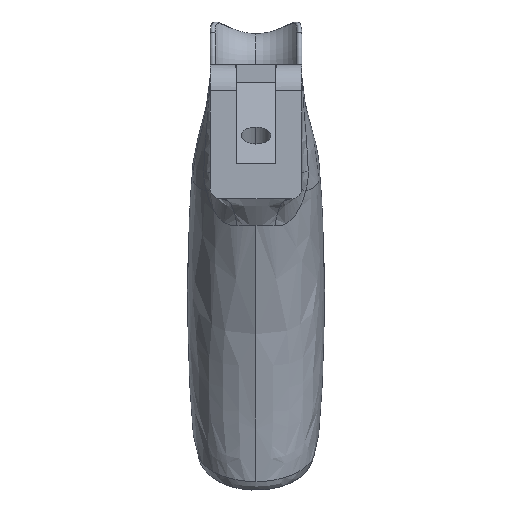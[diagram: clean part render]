
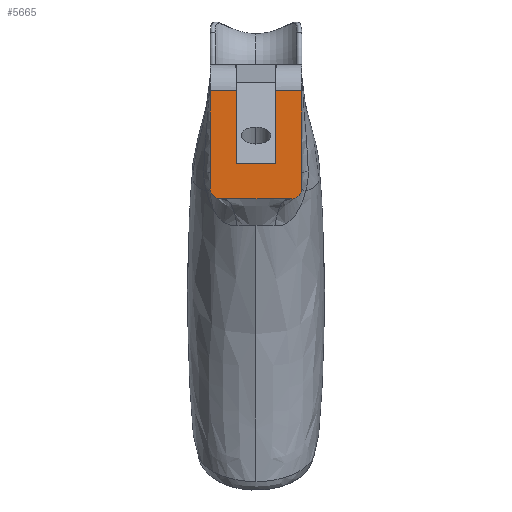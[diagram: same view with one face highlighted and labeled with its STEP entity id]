
A CAD part, top view. The second image highlights one B-rep face of the part: STEP entity #5665.
In plain terms, the highlighted planar face has unit normal (0, 0, 1).
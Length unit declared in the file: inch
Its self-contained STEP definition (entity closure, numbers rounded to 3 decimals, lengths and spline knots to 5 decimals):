
#47 = VERTEX_POINT ( 'NONE', #6501 ) ;
#377 = ORIENTED_EDGE ( 'NONE', *, *, #3790, .T. ) ;
#420 = DIRECTION ( 'NONE',  ( 0., 0., -1. ) ) ;
#441 = CARTESIAN_POINT ( 'NONE',  ( 0.1875, -0.25, 0. ) ) ;
#486 = CARTESIAN_POINT ( 'NONE',  ( 0.4375, -1.2789, 0. ) ) ;
#601 = VERTEX_POINT ( 'NONE', #441 ) ;
#726 = CARTESIAN_POINT ( 'NONE',  ( -0.3375, -1.2789, 0. ) ) ;
#776 = EDGE_CURVE ( 'NONE', #3794, #4979, #1841, .T. ) ;
#785 = EDGE_CURVE ( 'NONE', #3794, #4876, #6398, .T. ) ;
#873 = VERTEX_POINT ( 'NONE', #4419 ) ;
#920 = EDGE_LOOP ( 'NONE', ( #2350, #3677, #5511, #1936, #3274, #3456, #5523, #2167, #377, #1295 ) ) ;
#968 = CARTESIAN_POINT ( 'NONE',  ( 0.4375, -0.25, 0. ) ) ;
#1002 = LINE ( 'NONE', #2136, #7132 ) ;
#1037 = CARTESIAN_POINT ( 'NONE',  ( -0.1875, -0.94, 0. ) ) ;
#1239 = CARTESIAN_POINT ( 'NONE',  ( 0.4375, -0.25, 0. ) ) ;
#1260 = CARTESIAN_POINT ( 'NONE',  ( 0.4375, -1.1789, 0. ) ) ;
#1295 = ORIENTED_EDGE ( 'NONE', *, *, #1560, .T. ) ;
#1520 = VERTEX_POINT ( 'NONE', #6981 ) ;
#1556 = VERTEX_POINT ( 'NONE', #4774 ) ;
#1560 = EDGE_CURVE ( 'NONE', #1520, #873, #6086, .T. ) ;
#1602 = PLANE ( 'NONE',  #4865 ) ;
#1802 = CARTESIAN_POINT ( 'NONE',  ( -0.1875, -0.25, 0. ) ) ;
#1841 = LINE ( 'NONE', #1802, #2324 ) ;
#1936 = ORIENTED_EDGE ( 'NONE', *, *, #6627, .T. ) ;
#1941 = CARTESIAN_POINT ( 'NONE',  ( -0.4375, -1.1789, 0. ) ) ;
#2026 = EDGE_CURVE ( 'NONE', #2420, #3248, #6526, .T. ) ;
#2128 = LINE ( 'NONE', #486, #2840 ) ;
#2136 = CARTESIAN_POINT ( 'NONE',  ( 0.1875, -0.25, 0. ) ) ;
#2167 = ORIENTED_EDGE ( 'NONE', *, *, #785, .T. ) ;
#2244 = CARTESIAN_POINT ( 'NONE',  ( -0.1875, -0.94, 0. ) ) ;
#2324 = VECTOR ( 'NONE', #4114, 39.37008 ) ;
#2350 = ORIENTED_EDGE ( 'NONE', *, *, #6909, .F. ) ;
#2420 = VERTEX_POINT ( 'NONE', #5947 ) ;
#2421 = CARTESIAN_POINT ( 'NONE',  ( -0.1875, -0.25, 0. ) ) ;
#2707 = DIRECTION ( 'NONE',  ( 0., 1., 0. ) ) ;
#2774 = EDGE_CURVE ( 'NONE', #601, #1556, #1002, .T. ) ;
#2840 = VECTOR ( 'NONE', #3906, 39.37008 ) ;
#2917 = EDGE_CURVE ( 'NONE', #47, #3248, #5306, .T. ) ;
#3248 = VERTEX_POINT ( 'NONE', #1260 ) ;
#3274 = ORIENTED_EDGE ( 'NONE', *, *, #2774, .T. ) ;
#3319 = DIRECTION ( 'NONE',  ( 1., 0., 0. ) ) ;
#3456 = ORIENTED_EDGE ( 'NONE', *, *, #3643, .F. ) ;
#3549 = VECTOR ( 'NONE', #5501, 39.37008 ) ;
#3643 = EDGE_CURVE ( 'NONE', #4979, #1556, #5673, .T. ) ;
#3677 = ORIENTED_EDGE ( 'NONE', *, *, #2917, .T. ) ;
#3679 = CARTESIAN_POINT ( 'NONE',  ( 0.4375, -0.25, 0. ) ) ;
#3790 = EDGE_CURVE ( 'NONE', #4876, #1520, #4724, .T. ) ;
#3794 = VERTEX_POINT ( 'NONE', #2421 ) ;
#3906 = DIRECTION ( 'NONE',  ( -1., 0., 0. ) ) ;
#4021 = VECTOR ( 'NONE', #5195, 39.37008 ) ;
#4074 = CARTESIAN_POINT ( 'NONE',  ( 0.4375, -1.1789, 0. ) ) ;
#4114 = DIRECTION ( 'NONE',  ( 0., -1., 0. ) ) ;
#4252 = CARTESIAN_POINT ( 'NONE',  ( -0.4375, -1.2789, 0. ) ) ;
#4334 = CARTESIAN_POINT ( 'NONE',  ( 0.4375, -0.25, 0. ) ) ;
#4419 = CARTESIAN_POINT ( 'NONE',  ( -0.3375, -1.2789, 0. ) ) ;
#4580 = CARTESIAN_POINT ( 'NONE',  ( -0.4375, -0.25, 0. ) ) ;
#4622 = VECTOR ( 'NONE', #5485, 39.37008 ) ;
#4630 = CARTESIAN_POINT ( 'NONE',  ( 0.3375, -1.2789, 0. ) ) ;
#4724 = LINE ( 'NONE', #4580, #7269 ) ;
#4774 = CARTESIAN_POINT ( 'NONE',  ( 0.1875, -0.94, 0. ) ) ;
#4865 = AXIS2_PLACEMENT_3D ( 'NONE', #968, #420, #2707 ) ;
#4876 = VERTEX_POINT ( 'NONE', #5573 ) ;
#4979 = VERTEX_POINT ( 'NONE', #1037 ) ;
#5195 = DIRECTION ( 'NONE',  ( -1., 0., 0. ) ) ;
#5306 =( BOUNDED_CURVE ( )  B_SPLINE_CURVE ( 2, ( #4630, #6916, #4074 ),
 .UNSPECIFIED., .F., .F. ) 
 B_SPLINE_CURVE_WITH_KNOTS ( ( 3, 3 ),
 ( 0., 0.00397 ),
 .UNSPECIFIED. ) 
 CURVE ( )  GEOMETRIC_REPRESENTATION_ITEM ( )  RATIONAL_B_SPLINE_CURVE ( ( 1., 0.707, 1. ) ) 
 REPRESENTATION_ITEM ( '' )  );
#5485 = DIRECTION ( 'NONE',  ( 0., -1., 0. ) ) ;
#5501 = DIRECTION ( 'NONE',  ( -1., 0., 0. ) ) ;
#5511 = ORIENTED_EDGE ( 'NONE', *, *, #2026, .F. ) ;
#5523 = ORIENTED_EDGE ( 'NONE', *, *, #776, .F. ) ;
#5573 = CARTESIAN_POINT ( 'NONE',  ( -0.4375, -0.25, 0. ) ) ;
#5665 = ADVANCED_FACE ( 'NONE', ( #6127 ), #1602, .F. ) ;
#5673 = LINE ( 'NONE', #2244, #6662 ) ;
#5947 = CARTESIAN_POINT ( 'NONE',  ( 0.4375, -0.25, 0. ) ) ;
#6086 =( BOUNDED_CURVE ( )  B_SPLINE_CURVE ( 2, ( #1941, #4252, #726 ),
 .UNSPECIFIED., .F., .F. ) 
 B_SPLINE_CURVE_WITH_KNOTS ( ( 3, 3 ),
 ( 0., 0.00397 ),
 .UNSPECIFIED. ) 
 CURVE ( )  GEOMETRIC_REPRESENTATION_ITEM ( )  RATIONAL_B_SPLINE_CURVE ( ( 1., 0.707, 1. ) ) 
 REPRESENTATION_ITEM ( '' )  );
#6127 = FACE_OUTER_BOUND ( 'NONE', #920, .T. ) ;
#6163 = DIRECTION ( 'NONE',  ( 0., -1., 0. ) ) ;
#6398 = LINE ( 'NONE', #1239, #4021 ) ;
#6501 = CARTESIAN_POINT ( 'NONE',  ( 0.3375, -1.2789, 0. ) ) ;
#6526 = LINE ( 'NONE', #3679, #4622 ) ;
#6574 = LINE ( 'NONE', #4334, #3549 ) ;
#6627 = EDGE_CURVE ( 'NONE', #2420, #601, #6574, .T. ) ;
#6662 = VECTOR ( 'NONE', #3319, 39.37008 ) ;
#6904 = DIRECTION ( 'NONE',  ( 0., -1., 0. ) ) ;
#6909 = EDGE_CURVE ( 'NONE', #47, #873, #2128, .T. ) ;
#6916 = CARTESIAN_POINT ( 'NONE',  ( 0.4375, -1.2789, 0. ) ) ;
#6981 = CARTESIAN_POINT ( 'NONE',  ( -0.4375, -1.1789, 0. ) ) ;
#7132 = VECTOR ( 'NONE', #6163, 39.37008 ) ;
#7269 = VECTOR ( 'NONE', #6904, 39.37008 ) ;
